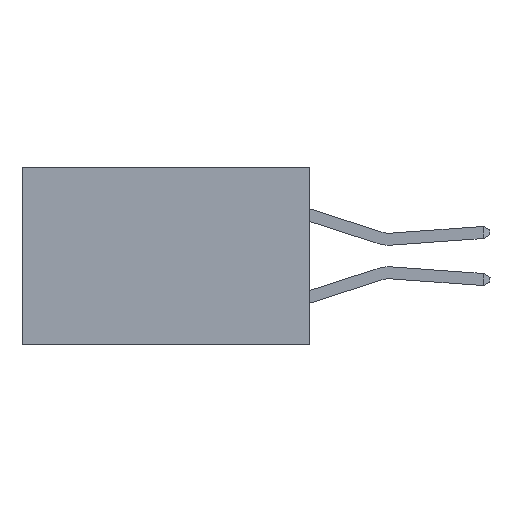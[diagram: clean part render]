
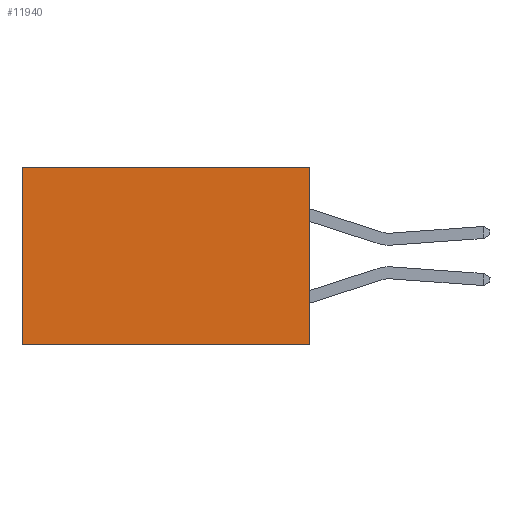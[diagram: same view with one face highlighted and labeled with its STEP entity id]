
A CAD part, left-side view. The second image highlights one B-rep face of the part: STEP entity #11940.
In plain terms, the highlighted planar face has unit normal (-1, 0, 0).
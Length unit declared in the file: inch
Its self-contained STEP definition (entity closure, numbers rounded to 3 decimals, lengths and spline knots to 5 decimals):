
#110 = ORIENTED_EDGE ( 'NONE', *, *, #1249, .F. ) ;
#248 = CARTESIAN_POINT ( 'NONE',  ( 0.298, 0., 0. ) ) ;
#702 = CARTESIAN_POINT ( 'NONE',  ( 0.298, 0., 0. ) ) ;
#1171 = PLANE ( 'NONE',  #13291 ) ;
#1249 = EDGE_CURVE ( 'NONE', #16510, #5122, #16989, .T. ) ;
#1289 = ORIENTED_EDGE ( 'NONE', *, *, #15583, .T. ) ;
#1794 = DIRECTION ( 'NONE',  ( 0., 1., 0. ) ) ;
#2375 = CARTESIAN_POINT ( 'NONE',  ( 0.298, 0.6, -0.37 ) ) ;
#2537 = CARTESIAN_POINT ( 'NONE',  ( 0.298, 0., 0. ) ) ;
#3604 = DIRECTION ( 'NONE',  ( 0., 0., -1. ) ) ;
#3908 = DIRECTION ( 'NONE',  ( 1., 0., 0. ) ) ;
#4184 = CARTESIAN_POINT ( 'NONE',  ( 0.298, 0., -0.37 ) ) ;
#4839 = EDGE_CURVE ( 'NONE', #16535, #6130, #9990, .T. ) ;
#5122 = VERTEX_POINT ( 'NONE', #4184 ) ;
#5889 = DIRECTION ( 'NONE',  ( 0., 0., -1. ) ) ;
#6130 = VERTEX_POINT ( 'NONE', #2375 ) ;
#6458 = CARTESIAN_POINT ( 'NONE',  ( 0.298, 0., -0.37 ) ) ;
#6701 = DIRECTION ( 'NONE',  ( 0., 0., -1. ) ) ;
#7480 = VECTOR ( 'NONE', #3604, 39.37008 ) ;
#7648 = ORIENTED_EDGE ( 'NONE', *, *, #13953, .F. ) ;
#7912 = LINE ( 'NONE', #6458, #12156 ) ;
#8862 = CARTESIAN_POINT ( 'NONE',  ( 0.298, 0.6, 0. ) ) ;
#9893 = FACE_OUTER_BOUND ( 'NONE', #12933, .T. ) ;
#9990 = LINE ( 'NONE', #12955, #14205 ) ;
#11833 = DIRECTION ( 'NONE',  ( 0., 1., 0. ) ) ;
#11887 = VECTOR ( 'NONE', #1794, 39.37008 ) ;
#11940 = ADVANCED_FACE ( 'NONE', ( #9893 ), #1171, .F. ) ;
#12156 = VECTOR ( 'NONE', #11833, 39.37008 ) ;
#12933 = EDGE_LOOP ( 'NONE', ( #14597, #7648, #110, #1289 ) ) ;
#12955 = CARTESIAN_POINT ( 'NONE',  ( 0.298, 0.6, 0. ) ) ;
#13291 = AXIS2_PLACEMENT_3D ( 'NONE', #2537, #3908, #6701 ) ;
#13953 = EDGE_CURVE ( 'NONE', #5122, #6130, #7912, .T. ) ;
#14205 = VECTOR ( 'NONE', #5889, 39.37008 ) ;
#14371 = CARTESIAN_POINT ( 'NONE',  ( 0.298, 0., 0. ) ) ;
#14597 = ORIENTED_EDGE ( 'NONE', *, *, #4839, .T. ) ;
#15497 = LINE ( 'NONE', #248, #11887 ) ;
#15583 = EDGE_CURVE ( 'NONE', #16510, #16535, #15497, .T. ) ;
#16510 = VERTEX_POINT ( 'NONE', #702 ) ;
#16535 = VERTEX_POINT ( 'NONE', #8862 ) ;
#16989 = LINE ( 'NONE', #14371, #7480 ) ;
